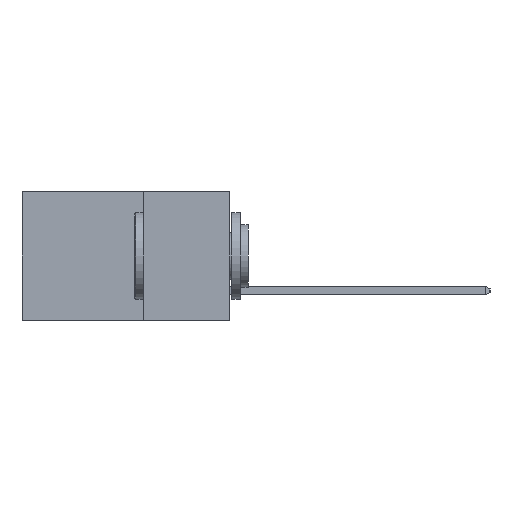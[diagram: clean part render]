
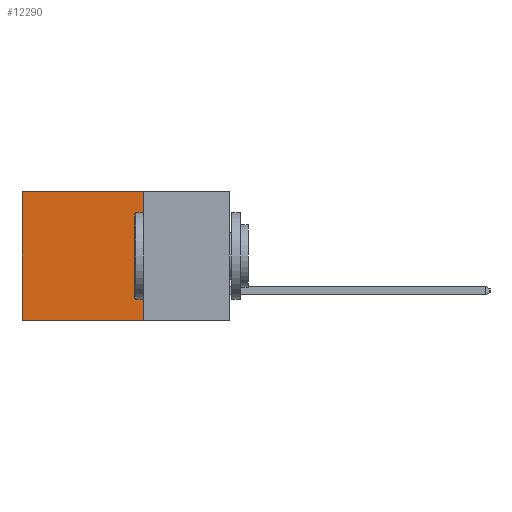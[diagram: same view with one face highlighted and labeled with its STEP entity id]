
A CAD part, left-side view. The second image highlights one B-rep face of the part: STEP entity #12290.
In plain terms, the highlighted planar face has unit normal (-1, 0, 0).
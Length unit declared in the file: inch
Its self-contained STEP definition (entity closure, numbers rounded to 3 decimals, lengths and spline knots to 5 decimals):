
#235 = LINE ( 'NONE', #2913, #21190 ) ;
#482 = EDGE_CURVE ( 'NONE', #12593, #18297, #16167, .T. ) ;
#807 = ORIENTED_EDGE ( 'NONE', *, *, #11807, .T. ) ;
#1765 = LINE ( 'NONE', #5265, #10020 ) ;
#2176 = VERTEX_POINT ( 'NONE', #8904 ) ;
#2913 = CARTESIAN_POINT ( 'NONE',  ( 0.298, 0.6, 0. ) ) ;
#3559 = ORIENTED_EDGE ( 'NONE', *, *, #482, .F. ) ;
#3587 = CARTESIAN_POINT ( 'NONE',  ( 0.298, 0.6, 0. ) ) ;
#5265 = CARTESIAN_POINT ( 'NONE',  ( 0.298, 0.25, 0. ) ) ;
#6550 = DIRECTION ( 'NONE',  ( 0., 0., -1. ) ) ;
#6914 = DIRECTION ( 'NONE',  ( 0., 1., 0. ) ) ;
#7737 = EDGE_CURVE ( 'NONE', #18297, #2176, #11873, .T. ) ;
#7911 = VECTOR ( 'NONE', #16446, 39.37008 ) ;
#8732 = ORIENTED_EDGE ( 'NONE', *, *, #7737, .F. ) ;
#8904 = CARTESIAN_POINT ( 'NONE',  ( 0.298, 0.6, -0.37 ) ) ;
#8993 = CARTESIAN_POINT ( 'NONE',  ( 0.298, 0.25, -0.37 ) ) ;
#9922 = VERTEX_POINT ( 'NONE', #3587 ) ;
#10020 = VECTOR ( 'NONE', #6914, 39.37008 ) ;
#10831 = VECTOR ( 'NONE', #18586, 39.37008 ) ;
#10993 = EDGE_CURVE ( 'NONE', #9922, #2176, #235, .T. ) ;
#11435 = AXIS2_PLACEMENT_3D ( 'NONE', #14739, #16424, #6550 ) ;
#11807 = EDGE_CURVE ( 'NONE', #12593, #9922, #1765, .T. ) ;
#11873 = LINE ( 'NONE', #18510, #10831 ) ;
#12290 = ADVANCED_FACE ( 'NONE', ( #17723 ), #19707, .F. ) ;
#12593 = VERTEX_POINT ( 'NONE', #16864 ) ;
#14739 = CARTESIAN_POINT ( 'NONE',  ( 0.298, 0.25, 0. ) ) ;
#16167 = LINE ( 'NONE', #16422, #7911 ) ;
#16422 = CARTESIAN_POINT ( 'NONE',  ( 0.298, 0.25, 0. ) ) ;
#16424 = DIRECTION ( 'NONE',  ( 1., 0., 0. ) ) ;
#16446 = DIRECTION ( 'NONE',  ( 0., 0., -1. ) ) ;
#16864 = CARTESIAN_POINT ( 'NONE',  ( 0.298, 0.25, 0. ) ) ;
#17723 = FACE_OUTER_BOUND ( 'NONE', #20322, .T. ) ;
#18297 = VERTEX_POINT ( 'NONE', #8993 ) ;
#18510 = CARTESIAN_POINT ( 'NONE',  ( 0.298, 0.25, -0.37 ) ) ;
#18522 = ORIENTED_EDGE ( 'NONE', *, *, #10993, .T. ) ;
#18586 = DIRECTION ( 'NONE',  ( 0., 1., 0. ) ) ;
#19451 = DIRECTION ( 'NONE',  ( 0., 0., -1. ) ) ;
#19707 = PLANE ( 'NONE',  #11435 ) ;
#20322 = EDGE_LOOP ( 'NONE', ( #18522, #8732, #3559, #807 ) ) ;
#21190 = VECTOR ( 'NONE', #19451, 39.37008 ) ;
